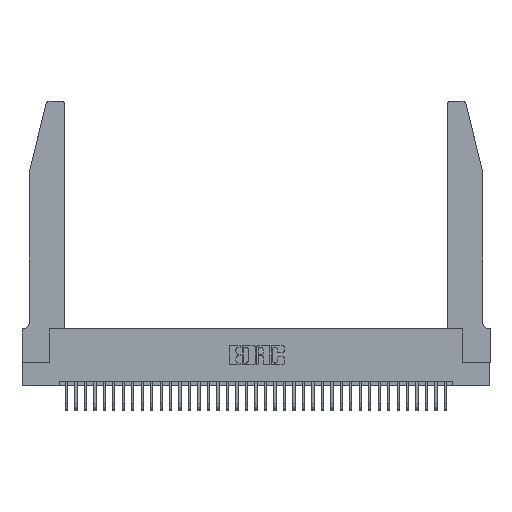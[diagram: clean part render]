
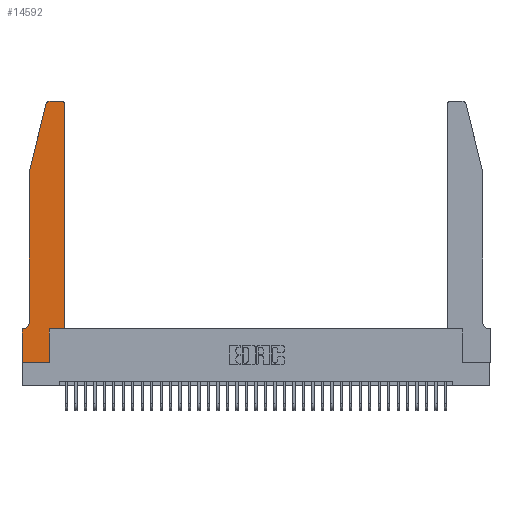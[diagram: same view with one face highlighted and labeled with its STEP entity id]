
A CAD part, top view. The second image highlights one B-rep face of the part: STEP entity #14592.
In plain terms, the highlighted planar face has unit normal (0, 0, 1).
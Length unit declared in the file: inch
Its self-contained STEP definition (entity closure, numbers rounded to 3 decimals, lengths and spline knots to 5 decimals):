
#321 = DIRECTION ( 'NONE',  ( 1., 0., 0. ) ) ;
#535 = ORIENTED_EDGE ( 'NONE', *, *, #4140, .T. ) ;
#670 = AXIS2_PLACEMENT_3D ( 'NONE', #20038, #3387, #22799 ) ;
#1233 = DIRECTION ( 'NONE',  ( 0., 0., -1. ) ) ;
#1272 = PLANE ( 'NONE',  #35722 ) ;
#1397 = DIRECTION ( 'NONE',  ( 1., 0., 0. ) ) ;
#1445 = ORIENTED_EDGE ( 'NONE', *, *, #4348, .T. ) ;
#1517 = CARTESIAN_POINT ( 'NONE',  ( 0.2865, 0., 0.37 ) ) ;
#1784 = VERTEX_POINT ( 'NONE', #9646 ) ;
#2448 = CARTESIAN_POINT ( 'NONE',  ( 0., 0.35, 0.37 ) ) ;
#2655 = LINE ( 'NONE', #27090, #30392 ) ;
#2665 = CARTESIAN_POINT ( 'NONE',  ( 0.0755, 2., 0.37 ) ) ;
#2907 = ORIENTED_EDGE ( 'NONE', *, *, #22394, .T. ) ;
#3342 = CARTESIAN_POINT ( 'NONE',  ( 0., 0., 0.37 ) ) ;
#3387 = DIRECTION ( 'NONE',  ( 0., 0., 1. ) ) ;
#3554 = CARTESIAN_POINT ( 'NONE',  ( 0.0755, 0.35, 0.37 ) ) ;
#3920 = VERTEX_POINT ( 'NONE', #18583 ) ;
#4140 = EDGE_CURVE ( 'NONE', #5977, #6320, #9829, .T. ) ;
#4348 = EDGE_CURVE ( 'NONE', #1784, #20641, #4560, .T. ) ;
#4560 = LINE ( 'NONE', #18068, #17628 ) ;
#4610 = LINE ( 'NONE', #5486, #32311 ) ;
#4930 = ORIENTED_EDGE ( 'NONE', *, *, #31231, .T. ) ;
#4933 = CIRCLE ( 'NONE', #11194, 0.03 ) ;
#5486 = CARTESIAN_POINT ( 'NONE',  ( 0., 0., 0.37 ) ) ;
#5827 = VERTEX_POINT ( 'NONE', #27006 ) ;
#5977 = VERTEX_POINT ( 'NONE', #16740 ) ;
#6320 = VERTEX_POINT ( 'NONE', #1517 ) ;
#6599 = VERTEX_POINT ( 'NONE', #2448 ) ;
#6905 = VERTEX_POINT ( 'NONE', #17761 ) ;
#6991 = DIRECTION ( 'NONE',  ( -0.239, -0.971, 0. ) ) ;
#7202 = CARTESIAN_POINT ( 'NONE',  ( 0.4505, 2.72, 0.37 ) ) ;
#8178 = CARTESIAN_POINT ( 'NONE',  ( 0.0055, 0.35, 0.37 ) ) ;
#8584 = EDGE_CURVE ( 'NONE', #3920, #23332, #21676, .T. ) ;
#8804 = ORIENTED_EDGE ( 'NONE', *, *, #29409, .T. ) ;
#8918 = EDGE_CURVE ( 'NONE', #20641, #3920, #16913, .T. ) ;
#9031 = LINE ( 'NONE', #16978, #16445 ) ;
#9646 = CARTESIAN_POINT ( 'NONE',  ( 0.25487, 2.72718, 0.37 ) ) ;
#9829 = LINE ( 'NONE', #3342, #33565 ) ;
#9858 = VERTEX_POINT ( 'NONE', #20212 ) ;
#10201 = VECTOR ( 'NONE', #18663, 39.37008 ) ;
#11085 = DIRECTION ( 'NONE',  ( 0., -1., 0. ) ) ;
#11194 = AXIS2_PLACEMENT_3D ( 'NONE', #27786, #11239, #30554 ) ;
#11239 = DIRECTION ( 'NONE',  ( 0., 0., 1. ) ) ;
#11783 = DIRECTION ( 'NONE',  ( 1., 0., 0. ) ) ;
#12487 = CARTESIAN_POINT ( 'NONE',  ( 0., 0.35, 0.37 ) ) ;
#13204 = CARTESIAN_POINT ( 'NONE',  ( 0.2605, 2.75, 0.37 ) ) ;
#13492 = EDGE_LOOP ( 'NONE', ( #8804, #13812, #1445, #29323, #15808, #18656, #34822, #535, #4930, #15658, #2907, #25193 ) ) ;
#13812 = ORIENTED_EDGE ( 'NONE', *, *, #29607, .T. ) ;
#14335 = EDGE_CURVE ( 'NONE', #5827, #27915, #9031, .T. ) ;
#14592 = ADVANCED_FACE ( 'NONE', ( #21574 ), #1272, .T. ) ;
#14917 = EDGE_CURVE ( 'NONE', #6599, #5977, #4610, .T. ) ;
#15658 = ORIENTED_EDGE ( 'NONE', *, *, #14335, .T. ) ;
#15808 = ORIENTED_EDGE ( 'NONE', *, *, #8584, .T. ) ;
#16110 = DIRECTION ( 'NONE',  ( 0., 1., 0. ) ) ;
#16445 = VECTOR ( 'NONE', #321, 39.37008 ) ;
#16740 = CARTESIAN_POINT ( 'NONE',  ( 0., 0., 0.37 ) ) ;
#16913 = LINE ( 'NONE', #2665, #24247 ) ;
#16978 = CARTESIAN_POINT ( 'NONE',  ( 0.4505, 0.35, 0.37 ) ) ;
#17428 = DIRECTION ( 'NONE',  ( -1., 0., 0. ) ) ;
#17628 = VECTOR ( 'NONE', #6991, 39.37008 ) ;
#17761 = CARTESIAN_POINT ( 'NONE',  ( 0.4205, 2.75, 0.37 ) ) ;
#17893 = CARTESIAN_POINT ( 'NONE',  ( 0.0055, 0.42, 0.37 ) ) ;
#18059 = DIRECTION ( 'NONE',  ( 0., 0., 1. ) ) ;
#18068 = CARTESIAN_POINT ( 'NONE',  ( 0.0755, 2., 0.37 ) ) ;
#18583 = CARTESIAN_POINT ( 'NONE',  ( 0.0755, 0.42, 0.37 ) ) ;
#18656 = ORIENTED_EDGE ( 'NONE', *, *, #19861, .T. ) ;
#18663 = DIRECTION ( 'NONE',  ( -1., 0., 0. ) ) ;
#18896 = LINE ( 'NONE', #20577, #32634 ) ;
#19861 = EDGE_CURVE ( 'NONE', #23332, #6599, #28077, .T. ) ;
#20038 = CARTESIAN_POINT ( 'NONE',  ( 0.4205, 2.72, 0.37 ) ) ;
#20050 = VERTEX_POINT ( 'NONE', #7202 ) ;
#20212 = CARTESIAN_POINT ( 'NONE',  ( 0.284, 2.75, 0.37 ) ) ;
#20577 = CARTESIAN_POINT ( 'NONE',  ( 0.4505, 0.35, 0.37 ) ) ;
#20641 = VERTEX_POINT ( 'NONE', #20698 ) ;
#20650 = DIRECTION ( 'NONE',  ( -1., 0., 0. ) ) ;
#20698 = CARTESIAN_POINT ( 'NONE',  ( 0.0755, 2., 0.37 ) ) ;
#21574 = FACE_OUTER_BOUND ( 'NONE', #13492, .T. ) ;
#21623 = EDGE_CURVE ( 'NONE', #20050, #6905, #35741, .T. ) ;
#21676 = CIRCLE ( 'NONE', #25252, 0.07 ) ;
#22394 = EDGE_CURVE ( 'NONE', #27915, #20050, #18896, .T. ) ;
#22799 = DIRECTION ( 'NONE',  ( 1., 0., 0. ) ) ;
#23332 = VERTEX_POINT ( 'NONE', #8178 ) ;
#23373 = DIRECTION ( 'NONE',  ( 0., 1., 0. ) ) ;
#24169 = CARTESIAN_POINT ( 'NONE',  ( 0.4505, 0.35, 0.37 ) ) ;
#24247 = VECTOR ( 'NONE', #11085, 39.37008 ) ;
#24936 = LINE ( 'NONE', #13204, #10201 ) ;
#25193 = ORIENTED_EDGE ( 'NONE', *, *, #21623, .T. ) ;
#25252 = AXIS2_PLACEMENT_3D ( 'NONE', #17893, #1233, #20650 ) ;
#27006 = CARTESIAN_POINT ( 'NONE',  ( 0.2865, 0.35, 0.37 ) ) ;
#27090 = CARTESIAN_POINT ( 'NONE',  ( 0.2865, 0.35, 0.37 ) ) ;
#27786 = CARTESIAN_POINT ( 'NONE',  ( 0.284, 2.72, 0.37 ) ) ;
#27915 = VERTEX_POINT ( 'NONE', #24169 ) ;
#28077 = LINE ( 'NONE', #3554, #35383 ) ;
#29323 = ORIENTED_EDGE ( 'NONE', *, *, #8918, .T. ) ;
#29409 = EDGE_CURVE ( 'NONE', #6905, #9858, #24936, .T. ) ;
#29607 = EDGE_CURVE ( 'NONE', #9858, #1784, #4933, .T. ) ;
#30091 = DIRECTION ( 'NONE',  ( 0., -1., 0. ) ) ;
#30392 = VECTOR ( 'NONE', #16110, 39.37008 ) ;
#30554 = DIRECTION ( 'NONE',  ( 1., 0., 0. ) ) ;
#31231 = EDGE_CURVE ( 'NONE', #6320, #5827, #2655, .T. ) ;
#32311 = VECTOR ( 'NONE', #30091, 39.37008 ) ;
#32634 = VECTOR ( 'NONE', #23373, 39.37008 ) ;
#33565 = VECTOR ( 'NONE', #11783, 39.37008 ) ;
#34822 = ORIENTED_EDGE ( 'NONE', *, *, #14917, .T. ) ;
#35383 = VECTOR ( 'NONE', #17428, 39.37008 ) ;
#35722 = AXIS2_PLACEMENT_3D ( 'NONE', #12487, #18059, #1397 ) ;
#35741 = CIRCLE ( 'NONE', #670, 0.03 ) ;
